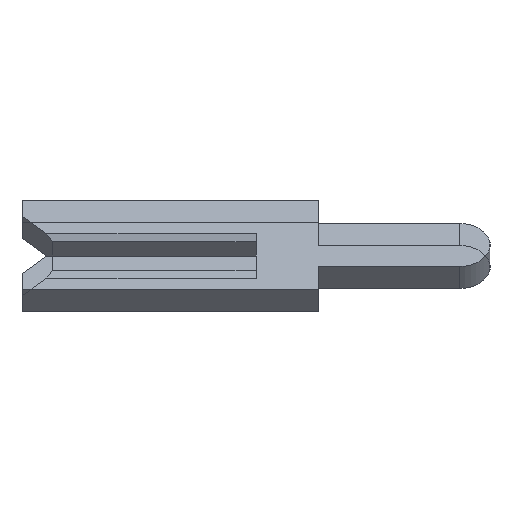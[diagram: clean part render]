
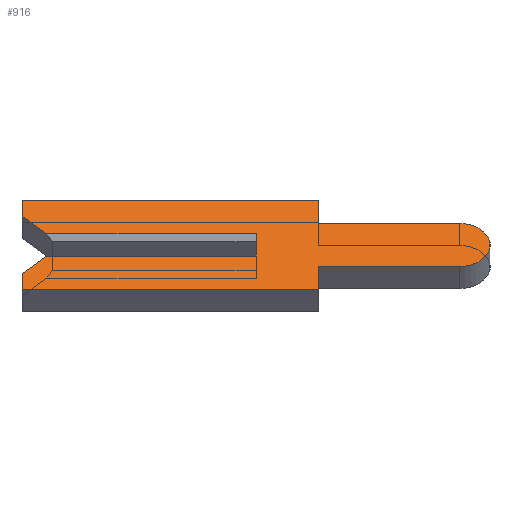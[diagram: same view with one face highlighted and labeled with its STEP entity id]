
A CAD part, left-side view. The second image highlights one B-rep face of the part: STEP entity #916.
In plain terms, the highlighted face is planar.
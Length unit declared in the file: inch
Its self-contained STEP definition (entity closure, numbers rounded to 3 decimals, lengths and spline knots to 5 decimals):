
#7 = VECTOR ( 'NONE', #1555, 39.37008 ) ;
#50 = EDGE_CURVE ( 'NONE', #3553, #3195, #732, .T. ) ;
#113 = CARTESIAN_POINT ( 'NONE',  ( -0.01, 0.15, 0.026 ) ) ;
#216 = EDGE_CURVE ( 'NONE', #2482, #605, #2532, .T. ) ;
#236 = EDGE_CURVE ( 'NONE', #2840, #1038, #826, .T. ) ;
#239 = CARTESIAN_POINT ( 'NONE',  ( -0.01, 0.15, -0.026 ) ) ;
#269 = VECTOR ( 'NONE', #1132, 39.37008 ) ;
#272 = CARTESIAN_POINT ( 'NONE',  ( -0.01, 0.134, 0.01 ) ) ;
#313 = LINE ( 'NONE', #3501, #2070 ) ;
#410 = LINE ( 'NONE', #710, #2977 ) ;
#530 = EDGE_CURVE ( 'NONE', #3590, #591, #972, .T. ) ;
#573 = PLANE ( 'NONE',  #1703 ) ;
#580 = ORIENTED_EDGE ( 'NONE', *, *, #3458, .F. ) ;
#586 = VERTEX_POINT ( 'NONE', #698 ) ;
#591 = VERTEX_POINT ( 'NONE', #1592 ) ;
#605 = VERTEX_POINT ( 'NONE', #2498 ) ;
#698 = CARTESIAN_POINT ( 'NONE',  ( -0.01, -0.1305, 0.0195 ) ) ;
#710 = CARTESIAN_POINT ( 'NONE',  ( -0.01, 0.15, -0.04 ) ) ;
#719 = CARTESIAN_POINT ( 'NONE',  ( -0.01, -0.1305, -0.0195 ) ) ;
#732 = LINE ( 'NONE', #3601, #7 ) ;
#733 = DIRECTION ( 'NONE',  ( 0., -1., 0. ) ) ;
#826 = LINE ( 'NONE', #3550, #2435 ) ;
#839 = CARTESIAN_POINT ( 'NONE',  ( -0.01, -0.1305, 0. ) ) ;
#846 = EDGE_CURVE ( 'NONE', #605, #3590, #1490, .T. ) ;
#879 = EDGE_CURVE ( 'NONE', #3644, #2840, #410, .T. ) ;
#900 = CARTESIAN_POINT ( 'NONE',  ( -0.01, 0.15, 0.01 ) ) ;
#916 = ADVANCED_FACE ( 'NONE', ( #3632 ), #573, .F. ) ;
#917 = CIRCLE ( 'NONE', #3252, 0.0195 ) ;
#972 = LINE ( 'NONE', #2458, #3302 ) ;
#1038 = VERTEX_POINT ( 'NONE', #239 ) ;
#1105 = VECTOR ( 'NONE', #1476, 39.37008 ) ;
#1110 = EDGE_CURVE ( 'NONE', #586, #3553, #917, .T. ) ;
#1115 = ORIENTED_EDGE ( 'NONE', *, *, #879, .F. ) ;
#1121 = CARTESIAN_POINT ( 'NONE',  ( -0.01, 0.134, -0.01 ) ) ;
#1132 = DIRECTION ( 'NONE',  ( 0., 0., -1. ) ) ;
#1274 = ORIENTED_EDGE ( 'NONE', *, *, #1110, .F. ) ;
#1301 = LINE ( 'NONE', #1502, #2651 ) ;
#1309 = DIRECTION ( 'NONE',  ( 0., 0., -1. ) ) ;
#1320 = CARTESIAN_POINT ( 'NONE',  ( -0.01, 0., 0.01 ) ) ;
#1452 = DIRECTION ( 'NONE',  ( 0., 0., -1. ) ) ;
#1476 = DIRECTION ( 'NONE',  ( 0., -1., 0. ) ) ;
#1490 = LINE ( 'NONE', #113, #2481 ) ;
#1502 = CARTESIAN_POINT ( 'NONE',  ( -0.01, -0.1305, -0.01 ) ) ;
#1555 = DIRECTION ( 'NONE',  ( 0., 1., 0. ) ) ;
#1592 = CARTESIAN_POINT ( 'NONE',  ( -0.01, -0.04, 0.04 ) ) ;
#1599 = CARTESIAN_POINT ( 'NONE',  ( -0.01, 0.15, 0.04 ) ) ;
#1612 = CARTESIAN_POINT ( 'NONE',  ( -0.01, -0.04, -0.04 ) ) ;
#1621 = VECTOR ( 'NONE', #1309, 39.37008 ) ;
#1632 = DIRECTION ( 'NONE',  ( 0., 0., 1. ) ) ;
#1636 = VERTEX_POINT ( 'NONE', #1121 ) ;
#1652 = EDGE_LOOP ( 'NONE', ( #2843, #3073, #3256, #2719, #3215, #1115, #580, #3026, #1274, #3541, #2983, #3624, #1806, #1817 ) ) ;
#1703 = AXIS2_PLACEMENT_3D ( 'NONE', #839, #3151, #1452 ) ;
#1773 = VERTEX_POINT ( 'NONE', #2872 ) ;
#1777 = EDGE_CURVE ( 'NONE', #591, #1773, #2116, .T. ) ;
#1806 = ORIENTED_EDGE ( 'NONE', *, *, #846, .F. ) ;
#1817 = ORIENTED_EDGE ( 'NONE', *, *, #216, .F. ) ;
#1824 = DIRECTION ( 'NONE',  ( 0., -0.707, 0.707 ) ) ;
#1884 = CARTESIAN_POINT ( 'NONE',  ( -0.01, -0.04, -0.0195 ) ) ;
#1899 = VECTOR ( 'NONE', #1824, 39.37008 ) ;
#1935 = DIRECTION ( 'NONE',  ( 1., 0., 0. ) ) ;
#2040 = EDGE_CURVE ( 'NONE', #2482, #3585, #2883, .T. ) ;
#2070 = VECTOR ( 'NONE', #3515, 39.37008 ) ;
#2116 = LINE ( 'NONE', #2583, #269 ) ;
#2139 = EDGE_CURVE ( 'NONE', #1636, #2214, #1301, .T. ) ;
#2202 = VECTOR ( 'NONE', #733, 39.37008 ) ;
#2214 = VERTEX_POINT ( 'NONE', #3534 ) ;
#2216 = EDGE_CURVE ( 'NONE', #2214, #3585, #313, .T. ) ;
#2318 = DIRECTION ( 'NONE',  ( 0., 1., 0. ) ) ;
#2382 = LINE ( 'NONE', #1612, #1621 ) ;
#2394 = CARTESIAN_POINT ( 'NONE',  ( -0.01, 0.15, -0.04 ) ) ;
#2435 = VECTOR ( 'NONE', #3270, 39.37008 ) ;
#2454 = CARTESIAN_POINT ( 'NONE',  ( -0.01, -0.04, 0.0195 ) ) ;
#2458 = CARTESIAN_POINT ( 'NONE',  ( -0.01, 0.15, 0.04 ) ) ;
#2481 = VECTOR ( 'NONE', #1632, 39.37008 ) ;
#2482 = VERTEX_POINT ( 'NONE', #272 ) ;
#2498 = CARTESIAN_POINT ( 'NONE',  ( -0.01, 0.15, 0.026 ) ) ;
#2532 = LINE ( 'NONE', #2974, #3536 ) ;
#2583 = CARTESIAN_POINT ( 'NONE',  ( -0.01, -0.04, 0.04 ) ) ;
#2591 = CARTESIAN_POINT ( 'NONE',  ( -0.01, -0.1305, 0. ) ) ;
#2601 = DIRECTION ( 'NONE',  ( 0., 0., -1. ) ) ;
#2627 = DIRECTION ( 'NONE',  ( 0., -1., 0. ) ) ;
#2651 = VECTOR ( 'NONE', #2627, 39.37008 ) ;
#2719 = ORIENTED_EDGE ( 'NONE', *, *, #2812, .F. ) ;
#2731 = CARTESIAN_POINT ( 'NONE',  ( -0.01, 0.1305, -0.0065 ) ) ;
#2770 = CARTESIAN_POINT ( 'NONE',  ( -0.01, -0.04, -0.04 ) ) ;
#2812 = EDGE_CURVE ( 'NONE', #1038, #1636, #3530, .T. ) ;
#2840 = VERTEX_POINT ( 'NONE', #2394 ) ;
#2843 = ORIENTED_EDGE ( 'NONE', *, *, #2040, .T. ) ;
#2872 = CARTESIAN_POINT ( 'NONE',  ( -0.01, -0.04, 0.0195 ) ) ;
#2883 = LINE ( 'NONE', #900, #1105 ) ;
#2974 = CARTESIAN_POINT ( 'NONE',  ( -0.01, 0.1305, 0.0065 ) ) ;
#2977 = VECTOR ( 'NONE', #2318, 39.37008 ) ;
#2983 = ORIENTED_EDGE ( 'NONE', *, *, #1777, .F. ) ;
#3014 = DIRECTION ( 'NONE',  ( 0., 0.707, 0.707 ) ) ;
#3026 = ORIENTED_EDGE ( 'NONE', *, *, #50, .F. ) ;
#3073 = ORIENTED_EDGE ( 'NONE', *, *, #2216, .F. ) ;
#3151 = DIRECTION ( 'NONE',  ( 1., 0., 0. ) ) ;
#3195 = VERTEX_POINT ( 'NONE', #1884 ) ;
#3215 = ORIENTED_EDGE ( 'NONE', *, *, #236, .F. ) ;
#3252 = AXIS2_PLACEMENT_3D ( 'NONE', #2591, #1935, #2601 ) ;
#3256 = ORIENTED_EDGE ( 'NONE', *, *, #2139, .F. ) ;
#3259 = EDGE_CURVE ( 'NONE', #1773, #586, #3264, .T. ) ;
#3264 = LINE ( 'NONE', #2454, #2202 ) ;
#3270 = DIRECTION ( 'NONE',  ( 0., 0., 1. ) ) ;
#3302 = VECTOR ( 'NONE', #3628, 39.37008 ) ;
#3458 = EDGE_CURVE ( 'NONE', #3195, #3644, #2382, .T. ) ;
#3501 = CARTESIAN_POINT ( 'NONE',  ( -0.01, 0., 0.0065 ) ) ;
#3515 = DIRECTION ( 'NONE',  ( 0., 0., 1. ) ) ;
#3530 = LINE ( 'NONE', #2731, #1899 ) ;
#3534 = CARTESIAN_POINT ( 'NONE',  ( -0.01, 0., -0.01 ) ) ;
#3536 = VECTOR ( 'NONE', #3014, 39.37008 ) ;
#3541 = ORIENTED_EDGE ( 'NONE', *, *, #3259, .F. ) ;
#3550 = CARTESIAN_POINT ( 'NONE',  ( -0.01, 0.15, -0.026 ) ) ;
#3553 = VERTEX_POINT ( 'NONE', #719 ) ;
#3585 = VERTEX_POINT ( 'NONE', #1320 ) ;
#3590 = VERTEX_POINT ( 'NONE', #1599 ) ;
#3601 = CARTESIAN_POINT ( 'NONE',  ( -0.01, -0.04, -0.0195 ) ) ;
#3624 = ORIENTED_EDGE ( 'NONE', *, *, #530, .F. ) ;
#3628 = DIRECTION ( 'NONE',  ( 0., -1., 0. ) ) ;
#3632 = FACE_OUTER_BOUND ( 'NONE', #1652, .T. ) ;
#3644 = VERTEX_POINT ( 'NONE', #2770 ) ;
